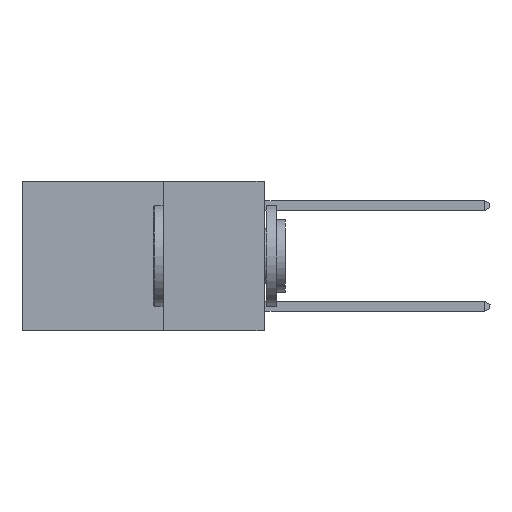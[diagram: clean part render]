
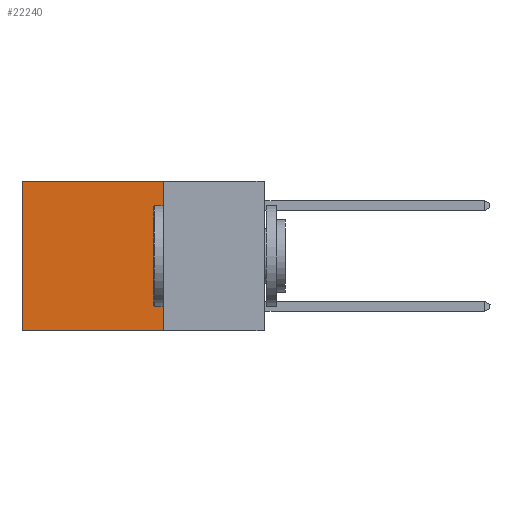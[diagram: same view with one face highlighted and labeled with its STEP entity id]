
A CAD part, left-side view. The second image highlights one B-rep face of the part: STEP entity #22240.
In plain terms, the highlighted planar face has unit normal (-1, 0, 0).
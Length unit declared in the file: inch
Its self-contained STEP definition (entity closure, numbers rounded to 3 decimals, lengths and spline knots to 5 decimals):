
#142 = EDGE_CURVE ( 'NONE', #2070, #6283, #20128, .T. ) ;
#655 = CARTESIAN_POINT ( 'NONE',  ( 0.2625, 0.25, 0. ) ) ;
#1023 = EDGE_LOOP ( 'NONE', ( #13044, #9229, #1732, #10231 ) ) ;
#1562 = EDGE_CURVE ( 'NONE', #8295, #6283, #10469, .T. ) ;
#1732 = ORIENTED_EDGE ( 'NONE', *, *, #21679, .F. ) ;
#2070 = VERTEX_POINT ( 'NONE', #11295 ) ;
#5033 = CARTESIAN_POINT ( 'NONE',  ( 0.2625, 0.25, 0. ) ) ;
#5560 = FACE_OUTER_BOUND ( 'NONE', #1023, .T. ) ;
#5593 = CARTESIAN_POINT ( 'NONE',  ( 0.2625, 0.25, 0. ) ) ;
#5815 = DIRECTION ( 'NONE',  ( 0., 0., -1. ) ) ;
#6076 = CARTESIAN_POINT ( 'NONE',  ( 0.2625, 0.6, 0. ) ) ;
#6084 = EDGE_CURVE ( 'NONE', #13813, #8295, #11986, .T. ) ;
#6283 = VERTEX_POINT ( 'NONE', #21969 ) ;
#7379 = DIRECTION ( 'NONE',  ( 0., 1., 0. ) ) ;
#8099 = AXIS2_PLACEMENT_3D ( 'NONE', #5033, #8626, #20928 ) ;
#8295 = VERTEX_POINT ( 'NONE', #22279 ) ;
#8626 = DIRECTION ( 'NONE',  ( 1., 0., 0. ) ) ;
#9229 = ORIENTED_EDGE ( 'NONE', *, *, #142, .F. ) ;
#10231 = ORIENTED_EDGE ( 'NONE', *, *, #6084, .T. ) ;
#10469 = LINE ( 'NONE', #6076, #19280 ) ;
#10661 = CARTESIAN_POINT ( 'NONE',  ( 0.2625, 0.25, 0. ) ) ;
#11295 = CARTESIAN_POINT ( 'NONE',  ( 0.2625, 0.25, -0.37 ) ) ;
#11408 = VECTOR ( 'NONE', #7379, 39.37008 ) ;
#11986 = LINE ( 'NONE', #5593, #11408 ) ;
#13044 = ORIENTED_EDGE ( 'NONE', *, *, #1562, .T. ) ;
#13813 = VERTEX_POINT ( 'NONE', #655 ) ;
#16051 = VECTOR ( 'NONE', #20869, 39.37008 ) ;
#19192 = PLANE ( 'NONE',  #8099 ) ;
#19280 = VECTOR ( 'NONE', #5815, 39.37008 ) ;
#20128 = LINE ( 'NONE', #20919, #16051 ) ;
#20764 = LINE ( 'NONE', #10661, #21832 ) ;
#20869 = DIRECTION ( 'NONE',  ( 0., 1., 0. ) ) ;
#20919 = CARTESIAN_POINT ( 'NONE',  ( 0.2625, 0.25, -0.37 ) ) ;
#20928 = DIRECTION ( 'NONE',  ( 0., 0., -1. ) ) ;
#21679 = EDGE_CURVE ( 'NONE', #13813, #2070, #20764, .T. ) ;
#21832 = VECTOR ( 'NONE', #22884, 39.37008 ) ;
#21969 = CARTESIAN_POINT ( 'NONE',  ( 0.2625, 0.6, -0.37 ) ) ;
#22240 = ADVANCED_FACE ( 'NONE', ( #5560 ), #19192, .F. ) ;
#22279 = CARTESIAN_POINT ( 'NONE',  ( 0.2625, 0.6, 0. ) ) ;
#22884 = DIRECTION ( 'NONE',  ( 0., 0., -1. ) ) ;
